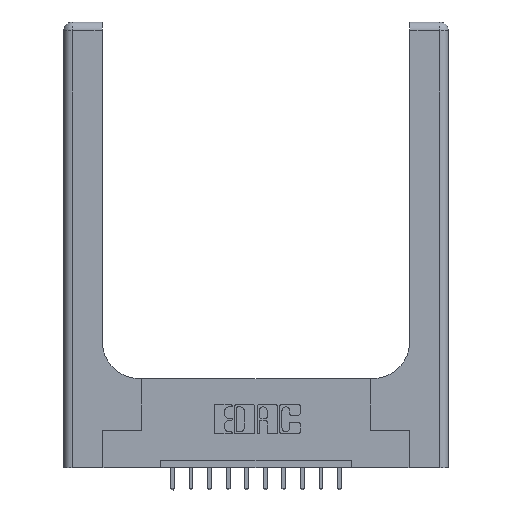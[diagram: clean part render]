
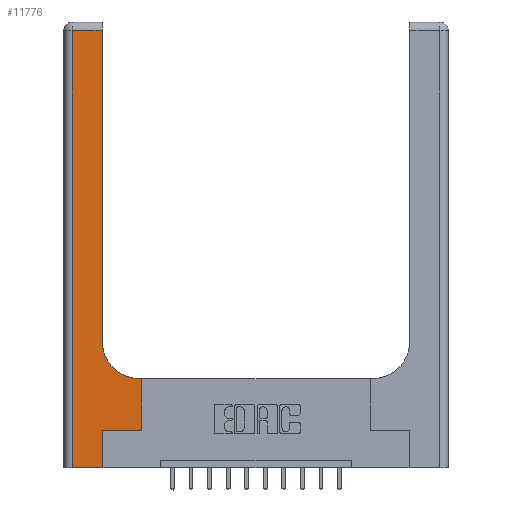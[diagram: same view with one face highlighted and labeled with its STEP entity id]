
A CAD part, top view. The second image highlights one B-rep face of the part: STEP entity #11776.
In plain terms, the highlighted planar face has unit normal (0, 0, 1).
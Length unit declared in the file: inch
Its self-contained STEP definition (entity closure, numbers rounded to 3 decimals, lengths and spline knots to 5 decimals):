
#359 = DIRECTION ( 'NONE',  ( 0., 1., 0. ) ) ;
#479 = LINE ( 'NONE', #10320, #15479 ) ;
#822 = VECTOR ( 'NONE', #6422, 39.37008 ) ;
#1452 = EDGE_CURVE ( 'NONE', #11523, #7608, #479, .T. ) ;
#1598 = LINE ( 'NONE', #13575, #8616 ) ;
#1621 = ORIENTED_EDGE ( 'NONE', *, *, #1766, .T. ) ;
#1766 = EDGE_CURVE ( 'NONE', #8048, #6685, #14565, .T. ) ;
#2204 = CARTESIAN_POINT ( 'NONE',  ( 0., 0., 0.37 ) ) ;
#2826 = CARTESIAN_POINT ( 'NONE',  ( 0.528, 0.25, 0.37 ) ) ;
#2971 = ORIENTED_EDGE ( 'NONE', *, *, #8357, .T. ) ;
#3446 = LINE ( 'NONE', #7383, #822 ) ;
#3784 = EDGE_CURVE ( 'NONE', #3797, #8018, #8443, .T. ) ;
#3797 = VERTEX_POINT ( 'NONE', #12833 ) ;
#4306 = VECTOR ( 'NONE', #14402, 39.37008 ) ;
#4568 = LINE ( 'NONE', #6144, #13943 ) ;
#5136 = LINE ( 'NONE', #14250, #12585 ) ;
#5160 = CARTESIAN_POINT ( 'NONE',  ( 0.06, 0., 0.37 ) ) ;
#5445 = DIRECTION ( 'NONE',  ( 0., -1., 0. ) ) ;
#5450 = LINE ( 'NONE', #2204, #4306 ) ;
#5484 = VERTEX_POINT ( 'NONE', #8555 ) ;
#6011 = DIRECTION ( 'NONE',  ( 0., 1., 0. ) ) ;
#6144 = CARTESIAN_POINT ( 'NONE',  ( 0., 2.94, 0.37 ) ) ;
#6199 = CARTESIAN_POINT ( 'NONE',  ( 0.06, 2.94, 0.37 ) ) ;
#6422 = DIRECTION ( 'NONE',  ( -1., 0., 0. ) ) ;
#6452 = CARTESIAN_POINT ( 'NONE',  ( 0.26, 0.85, 0.37 ) ) ;
#6685 = VERTEX_POINT ( 'NONE', #8557 ) ;
#6969 = EDGE_CURVE ( 'NONE', #8943, #8048, #1598, .T. ) ;
#7383 = CARTESIAN_POINT ( 'NONE',  ( 0.26, 0.6, 0.37 ) ) ;
#7608 = VERTEX_POINT ( 'NONE', #5160 ) ;
#7841 = CARTESIAN_POINT ( 'NONE',  ( 0.265, 0.25, 0.37 ) ) ;
#7966 = DIRECTION ( 'NONE',  ( 1., 0., 0. ) ) ;
#8018 = VERTEX_POINT ( 'NONE', #6452 ) ;
#8045 = DIRECTION ( 'NONE',  ( 0., 1., 0. ) ) ;
#8048 = VERTEX_POINT ( 'NONE', #12911 ) ;
#8357 = EDGE_CURVE ( 'NONE', #6685, #3797, #3446, .T. ) ;
#8443 = CIRCLE ( 'NONE', #8530, 0.25 ) ;
#8530 = AXIS2_PLACEMENT_3D ( 'NONE', #11421, #15339, #7966 ) ;
#8555 = CARTESIAN_POINT ( 'NONE',  ( 0.265, 0., 0.37 ) ) ;
#8557 = CARTESIAN_POINT ( 'NONE',  ( 0.528, 0.6, 0.37 ) ) ;
#8571 = DIRECTION ( 'NONE',  ( -1., 0., 0. ) ) ;
#8616 = VECTOR ( 'NONE', #9804, 39.37008 ) ;
#8720 = EDGE_CURVE ( 'NONE', #9686, #11523, #4568, .T. ) ;
#8943 = VERTEX_POINT ( 'NONE', #7841 ) ;
#9056 = EDGE_CURVE ( 'NONE', #5484, #8943, #5136, .T. ) ;
#9089 = VECTOR ( 'NONE', #6011, 39.37008 ) ;
#9110 = PLANE ( 'NONE',  #11812 ) ;
#9212 = DIRECTION ( 'NONE',  ( -1., 0., 0. ) ) ;
#9265 = LINE ( 'NONE', #9609, #9089 ) ;
#9609 = CARTESIAN_POINT ( 'NONE',  ( 0.26, 3., 0.37 ) ) ;
#9686 = VERTEX_POINT ( 'NONE', #14067 ) ;
#9788 = FACE_OUTER_BOUND ( 'NONE', #14944, .T. ) ;
#9804 = DIRECTION ( 'NONE',  ( 1., 0., 0. ) ) ;
#10320 = CARTESIAN_POINT ( 'NONE',  ( 0.06, 3., 0.37 ) ) ;
#10327 = EDGE_CURVE ( 'NONE', #8018, #9686, #9265, .T. ) ;
#11421 = CARTESIAN_POINT ( 'NONE',  ( 0.51, 0.85, 0.37 ) ) ;
#11523 = VERTEX_POINT ( 'NONE', #6199 ) ;
#11730 = DIRECTION ( 'NONE',  ( 0., 0., -1. ) ) ;
#11776 = ADVANCED_FACE ( 'NONE', ( #9788 ), #9110, .F. ) ;
#11812 = AXIS2_PLACEMENT_3D ( 'NONE', #15267, #11730, #9212 ) ;
#11816 = ORIENTED_EDGE ( 'NONE', *, *, #3784, .T. ) ;
#12361 = ORIENTED_EDGE ( 'NONE', *, *, #14965, .T. ) ;
#12376 = ORIENTED_EDGE ( 'NONE', *, *, #6969, .T. ) ;
#12415 = ORIENTED_EDGE ( 'NONE', *, *, #8720, .T. ) ;
#12585 = VECTOR ( 'NONE', #8045, 39.37008 ) ;
#12833 = CARTESIAN_POINT ( 'NONE',  ( 0.51, 0.6, 0.37 ) ) ;
#12911 = CARTESIAN_POINT ( 'NONE',  ( 0.528, 0.25, 0.37 ) ) ;
#13575 = CARTESIAN_POINT ( 'NONE',  ( 0.265, 0.25, 0.37 ) ) ;
#13943 = VECTOR ( 'NONE', #8571, 39.37008 ) ;
#14014 = VECTOR ( 'NONE', #359, 39.37008 ) ;
#14067 = CARTESIAN_POINT ( 'NONE',  ( 0.26, 2.94, 0.37 ) ) ;
#14250 = CARTESIAN_POINT ( 'NONE',  ( 0.265, 0., 0.37 ) ) ;
#14338 = ORIENTED_EDGE ( 'NONE', *, *, #9056, .T. ) ;
#14402 = DIRECTION ( 'NONE',  ( 1., 0., 0. ) ) ;
#14487 = ORIENTED_EDGE ( 'NONE', *, *, #10327, .T. ) ;
#14565 = LINE ( 'NONE', #2826, #14014 ) ;
#14944 = EDGE_LOOP ( 'NONE', ( #14487, #12415, #15628, #12361, #14338, #12376, #1621, #2971, #11816 ) ) ;
#14965 = EDGE_CURVE ( 'NONE', #7608, #5484, #5450, .T. ) ;
#15267 = CARTESIAN_POINT ( 'NONE',  ( 0., 3., 0.37 ) ) ;
#15339 = DIRECTION ( 'NONE',  ( 0., 0., -1. ) ) ;
#15479 = VECTOR ( 'NONE', #5445, 39.37008 ) ;
#15628 = ORIENTED_EDGE ( 'NONE', *, *, #1452, .T. ) ;
